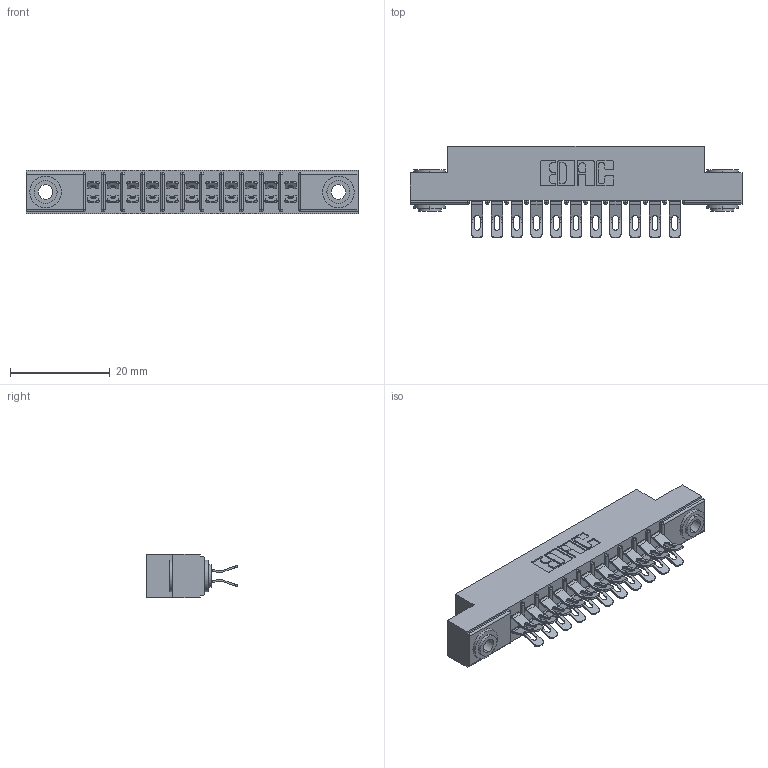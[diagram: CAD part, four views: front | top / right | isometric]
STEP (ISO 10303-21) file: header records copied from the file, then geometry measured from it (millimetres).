
FILE_DESCRIPTION (( 'STEP AP203' ), '1' );
FILE_NAME ('305-022-555-203.STEP', '2019-09-09T13:45:34', ( '' ), ( '' ), 'SwSTEP 2.0', 'SolidWorks 2016', '' );
FILE_SCHEMA (( 'CONFIG_CONTROL_DESIGN' ));
Length unit declared in the file: inch
Products named in the file (4): 345-250-002_345-250-002-102; 305 Part_.156 Dia; 305-290-001_555; 305-022-555-203
Assembly tree (25 placements, depth 2):
  305-022-555-203
    305 Part_.156 Dia
    305-290-001_555  x22
    345-250-002_345-250-002-102  x2
Bounding box: 66.6 x 18.41 x 8.71 mm (x, y, z)
Volume: 4255.9 mm3; surface area: 8021.2 mm2
Topology: 25 solids, 25 shells, 1620 faces, 4773 edges, 3118 vertices
Faces by surface type: plane 796, cylinder 772, sphere 44, cone 8
Entity records: 17373 total; most frequent: CARTESIAN_POINT 2874, ORIENTED_EDGE 2830, DIRECTION 2815, EDGE_CURVE 1415, VECTOR 1081, LINE 1081, VERTEX_POINT 910, AXIS2_PLACEMENT_3D 867
